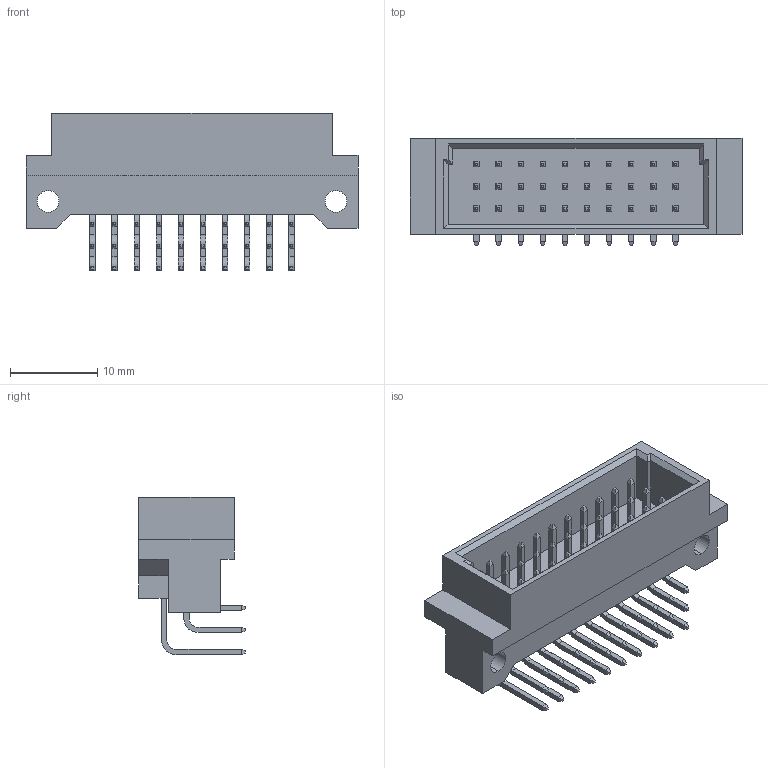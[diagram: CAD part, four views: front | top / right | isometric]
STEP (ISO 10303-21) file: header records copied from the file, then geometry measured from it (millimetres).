
FILE_DESCRIPTION (( 'STEP AP214' ), '1' );
FILE_NAME ('495-030-660-312.STEP', '2020-08-12T15:31:43', ( '' ), ( '' ), 'SwSTEP 2.0', 'SolidWorks 2020', '' );
FILE_SCHEMA (( 'AUTOMOTIVE_DESIGN' ));
Length unit declared in the file: millimetre
Products named in the file (5): 495-030-660-312; 495-290-2; 495-290-3; 495-290-1; 495 Part_30
Assembly tree (31 placements, depth 2):
  495-030-660-312
    495 Part_30
    495-290-1  x10
    495-290-2  x10
    495-290-3  x10
Bounding box: 38.1 x 12.27 x 18.05 mm (x, y, z)
Volume: 2675.9 mm3; surface area: 4286.9 mm2
Topology: 31 solids, 31 shells, 709 faces, 1688 edges, 1042 vertices
Faces by surface type: plane 645, cylinder 64
Entity records: 7412 total; most frequent: CARTESIAN_POINT 1259, ORIENTED_EDGE 1216, DIRECTION 1142, EDGE_CURVE 608, LINE 588, VECTOR 588, VERTEX_POINT 394, EDGE_LOOP 288
